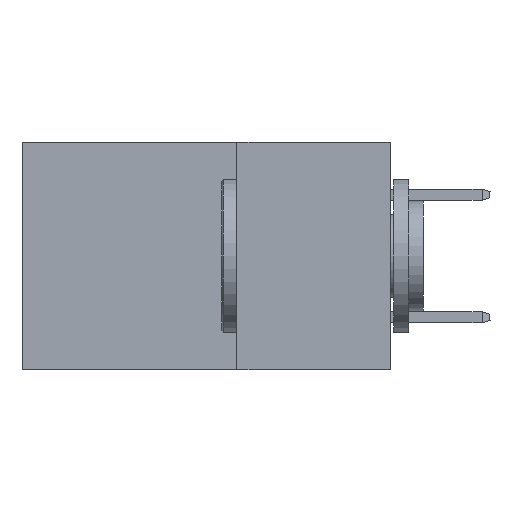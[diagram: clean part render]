
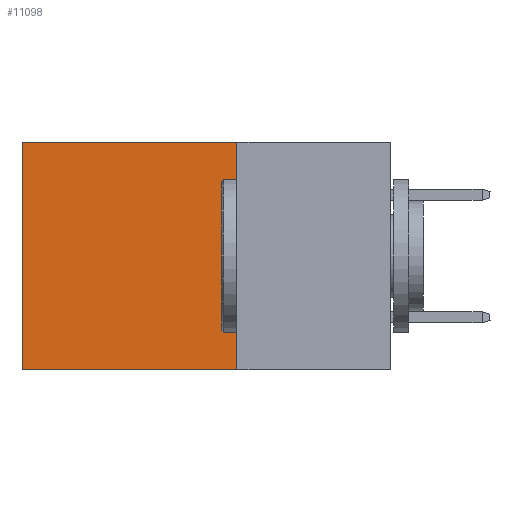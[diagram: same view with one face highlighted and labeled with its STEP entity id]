
A CAD part, left-side view. The second image highlights one B-rep face of the part: STEP entity #11098.
In plain terms, the highlighted planar face has unit normal (-1, 0, 0).
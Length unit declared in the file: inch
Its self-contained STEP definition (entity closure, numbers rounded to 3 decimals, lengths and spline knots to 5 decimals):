
#373 = CARTESIAN_POINT ( 'NONE',  ( 0.2875, 0.25, -0.37 ) ) ;
#581 = LINE ( 'NONE', #373, #16966 ) ;
#643 = PLANE ( 'NONE',  #1915 ) ;
#1349 = CARTESIAN_POINT ( 'NONE',  ( 0.2875, 0.6, 0. ) ) ;
#1685 = LINE ( 'NONE', #18830, #17108 ) ;
#1915 = AXIS2_PLACEMENT_3D ( 'NONE', #3631, #6632, #9721 ) ;
#2610 = EDGE_CURVE ( 'NONE', #19281, #2858, #16515, .T. ) ;
#2858 = VERTEX_POINT ( 'NONE', #5546 ) ;
#3003 = CARTESIAN_POINT ( 'NONE',  ( 0.2875, 0.6, 0. ) ) ;
#3631 = CARTESIAN_POINT ( 'NONE',  ( 0.2875, 0.25, 0. ) ) ;
#4951 = EDGE_CURVE ( 'NONE', #5320, #5211, #10334, .T. ) ;
#5211 = VERTEX_POINT ( 'NONE', #17622 ) ;
#5320 = VERTEX_POINT ( 'NONE', #1349 ) ;
#5546 = CARTESIAN_POINT ( 'NONE',  ( 0.2875, 0.25, -0.37 ) ) ;
#5743 = ORIENTED_EDGE ( 'NONE', *, *, #4951, .T. ) ;
#6148 = DIRECTION ( 'NONE',  ( 0., 0., -1. ) ) ;
#6311 = VECTOR ( 'NONE', #16470, 39.37008 ) ;
#6632 = DIRECTION ( 'NONE',  ( 1., 0., 0. ) ) ;
#7784 = EDGE_LOOP ( 'NONE', ( #5743, #17561, #8654, #10459 ) ) ;
#8095 = EDGE_CURVE ( 'NONE', #19281, #5320, #1685, .T. ) ;
#8335 = VECTOR ( 'NONE', #6148, 39.37008 ) ;
#8654 = ORIENTED_EDGE ( 'NONE', *, *, #2610, .F. ) ;
#9721 = DIRECTION ( 'NONE',  ( 0., 0., -1. ) ) ;
#10334 = LINE ( 'NONE', #3003, #6311 ) ;
#10459 = ORIENTED_EDGE ( 'NONE', *, *, #8095, .T. ) ;
#10917 = FACE_OUTER_BOUND ( 'NONE', #7784, .T. ) ;
#11098 = ADVANCED_FACE ( 'NONE', ( #10917 ), #643, .F. ) ;
#11446 = EDGE_CURVE ( 'NONE', #2858, #5211, #581, .T. ) ;
#13625 = CARTESIAN_POINT ( 'NONE',  ( 0.2875, 0.25, 0. ) ) ;
#13736 = DIRECTION ( 'NONE',  ( 0., 1., 0. ) ) ;
#16470 = DIRECTION ( 'NONE',  ( 0., 0., -1. ) ) ;
#16515 = LINE ( 'NONE', #13625, #8335 ) ;
#16966 = VECTOR ( 'NONE', #13736, 39.37008 ) ;
#17108 = VECTOR ( 'NONE', #17382, 39.37008 ) ;
#17382 = DIRECTION ( 'NONE',  ( 0., 1., 0. ) ) ;
#17561 = ORIENTED_EDGE ( 'NONE', *, *, #11446, .F. ) ;
#17622 = CARTESIAN_POINT ( 'NONE',  ( 0.2875, 0.6, -0.37 ) ) ;
#18059 = CARTESIAN_POINT ( 'NONE',  ( 0.2875, 0.25, 0. ) ) ;
#18830 = CARTESIAN_POINT ( 'NONE',  ( 0.2875, 0.25, 0. ) ) ;
#19281 = VERTEX_POINT ( 'NONE', #18059 ) ;
